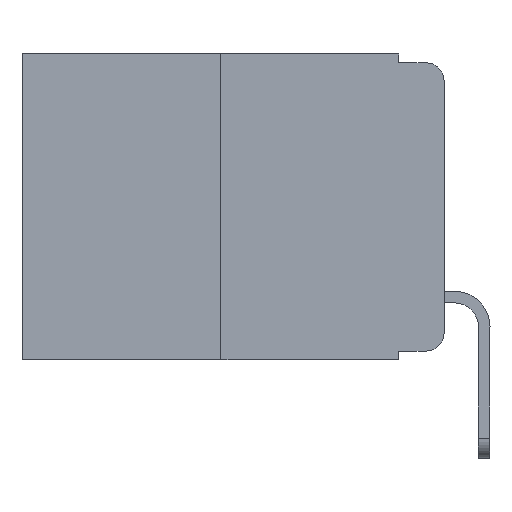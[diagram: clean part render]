
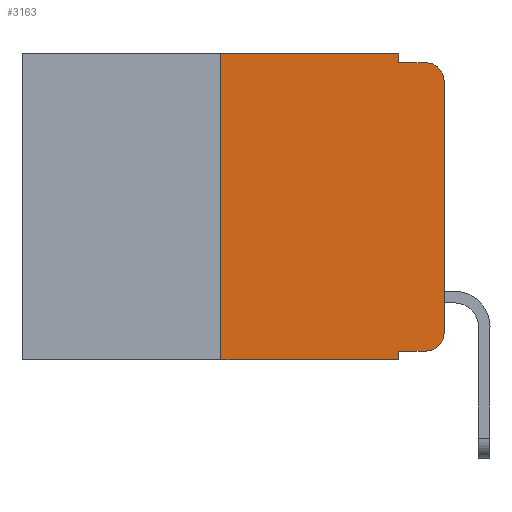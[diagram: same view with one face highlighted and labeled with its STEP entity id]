
A CAD part, left-side view. The second image highlights one B-rep face of the part: STEP entity #3163.
In plain terms, the highlighted planar face has unit normal (-1, 0, 0).
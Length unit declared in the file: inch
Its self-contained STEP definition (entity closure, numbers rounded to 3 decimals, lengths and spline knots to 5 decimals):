
#18 = DIRECTION ( 'NONE',  ( 0., 0., -1. ) ) ;
#445 = ORIENTED_EDGE ( 'NONE', *, *, #828, .F. ) ;
#467 = VERTEX_POINT ( 'NONE', #10976 ) ;
#617 = VERTEX_POINT ( 'NONE', #10006 ) ;
#828 = EDGE_CURVE ( 'NONE', #467, #3621, #6359, .T. ) ;
#1123 = EDGE_LOOP ( 'NONE', ( #1739, #3092, #2296, #1510, #1259, #13174, #13289, #445, #13529, #4531 ) ) ;
#1136 = VECTOR ( 'NONE', #7764, 39.37008 ) ;
#1208 = AXIS2_PLACEMENT_3D ( 'NONE', #9365, #3027, #10290 ) ;
#1259 = ORIENTED_EDGE ( 'NONE', *, *, #12937, .F. ) ;
#1381 = CARTESIAN_POINT ( 'NONE',  ( 0., 0.473, 0. ) ) ;
#1388 = FACE_OUTER_BOUND ( 'NONE', #1123, .T. ) ;
#1510 = ORIENTED_EDGE ( 'NONE', *, *, #7789, .F. ) ;
#1739 = ORIENTED_EDGE ( 'NONE', *, *, #2849, .T. ) ;
#1791 = LINE ( 'NONE', #5107, #4790 ) ;
#1983 = CARTESIAN_POINT ( 'NONE',  ( 0., 0.051, -0.01 ) ) ;
#2018 = EDGE_CURVE ( 'NONE', #2186, #3915, #1791, .T. ) ;
#2102 = EDGE_CURVE ( 'NONE', #617, #3561, #3253, .T. ) ;
#2186 = VERTEX_POINT ( 'NONE', #1983 ) ;
#2194 = DIRECTION ( 'NONE',  ( 0., 0., -1. ) ) ;
#2214 = DIRECTION ( 'NONE',  ( 0., -1., 0. ) ) ;
#2296 = ORIENTED_EDGE ( 'NONE', *, *, #2018, .F. ) ;
#2552 = DIRECTION ( 'NONE',  ( 0., 0., 1. ) ) ;
#2657 = EDGE_CURVE ( 'NONE', #6269, #3915, #12574, .T. ) ;
#2675 = DIRECTION ( 'NONE',  ( -1., 0., 0. ) ) ;
#2754 = EDGE_CURVE ( 'NONE', #10431, #3621, #8405, .T. ) ;
#2846 = LINE ( 'NONE', #9067, #4955 ) ;
#2849 = EDGE_CURVE ( 'NONE', #3561, #6269, #11659, .T. ) ;
#3027 = DIRECTION ( 'NONE',  ( -1., 0., 0. ) ) ;
#3092 = ORIENTED_EDGE ( 'NONE', *, *, #2657, .T. ) ;
#3163 = ADVANCED_FACE ( 'NONE', ( #1388 ), #7793, .F. ) ;
#3253 = CIRCLE ( 'NONE', #1208, 0.02 ) ;
#3314 = VECTOR ( 'NONE', #18, 39.37008 ) ;
#3561 = VERTEX_POINT ( 'NONE', #8453 ) ;
#3621 = VERTEX_POINT ( 'NONE', #13196 ) ;
#3915 = VERTEX_POINT ( 'NONE', #6934 ) ;
#4531 = ORIENTED_EDGE ( 'NONE', *, *, #2102, .T. ) ;
#4617 = LINE ( 'NONE', #11159, #9338 ) ;
#4790 = VECTOR ( 'NONE', #5153, 39.37008 ) ;
#4955 = VECTOR ( 'NONE', #6074, 39.37008 ) ;
#5042 = VERTEX_POINT ( 'NONE', #9473 ) ;
#5055 = CARTESIAN_POINT ( 'NONE',  ( 0., 0.25, 0. ) ) ;
#5107 = CARTESIAN_POINT ( 'NONE',  ( 0., 0.051, -0.01 ) ) ;
#5153 = DIRECTION ( 'NONE',  ( 0., -1., 0. ) ) ;
#5787 = CARTESIAN_POINT ( 'NONE',  ( 0., 0.473, 0. ) ) ;
#5897 = VERTEX_POINT ( 'NONE', #5055 ) ;
#6074 = DIRECTION ( 'NONE',  ( 0., -1., 0. ) ) ;
#6269 = VERTEX_POINT ( 'NONE', #8100 ) ;
#6359 = LINE ( 'NONE', #9684, #3314 ) ;
#6652 = VECTOR ( 'NONE', #2552, 39.37008 ) ;
#6779 = CARTESIAN_POINT ( 'NONE',  ( 0., 0.25, 0. ) ) ;
#6934 = CARTESIAN_POINT ( 'NONE',  ( 0., 0.02, -0.01 ) ) ;
#7169 = VECTOR ( 'NONE', #10117, 39.37008 ) ;
#7398 = DIRECTION ( 'NONE',  ( 0., 0., -1. ) ) ;
#7672 = LINE ( 'NONE', #6779, #1136 ) ;
#7764 = DIRECTION ( 'NONE',  ( 0., 0., 1. ) ) ;
#7789 = EDGE_CURVE ( 'NONE', #5042, #2186, #4617, .T. ) ;
#7793 = PLANE ( 'NONE',  #12513 ) ;
#7810 = CARTESIAN_POINT ( 'NONE',  ( 0., 0.473, -0.343 ) ) ;
#8100 = CARTESIAN_POINT ( 'NONE',  ( 0., 0., -0.03 ) ) ;
#8108 = VECTOR ( 'NONE', #2214, 39.37008 ) ;
#8405 = LINE ( 'NONE', #7810, #8108 ) ;
#8453 = CARTESIAN_POINT ( 'NONE',  ( 0., 0., -0.313 ) ) ;
#8757 = DIRECTION ( 'NONE',  ( 1., 0., 0. ) ) ;
#9067 = CARTESIAN_POINT ( 'NONE',  ( 0., 0.051, -0.333 ) ) ;
#9094 = CARTESIAN_POINT ( 'NONE',  ( 0., 0.02, -0.03 ) ) ;
#9244 = EDGE_CURVE ( 'NONE', #10431, #5897, #7672, .T. ) ;
#9338 = VECTOR ( 'NONE', #7398, 39.37008 ) ;
#9365 = CARTESIAN_POINT ( 'NONE',  ( 0., 0.02, -0.313 ) ) ;
#9473 = CARTESIAN_POINT ( 'NONE',  ( 0., 0.051, 0. ) ) ;
#9684 = CARTESIAN_POINT ( 'NONE',  ( 0., 0.051, 0. ) ) ;
#9976 = CARTESIAN_POINT ( 'NONE',  ( 0., 0., 0. ) ) ;
#10006 = CARTESIAN_POINT ( 'NONE',  ( 0., 0.02, -0.333 ) ) ;
#10057 = DIRECTION ( 'NONE',  ( 0., 0., -1. ) ) ;
#10117 = DIRECTION ( 'NONE',  ( 0., -1., 0. ) ) ;
#10290 = DIRECTION ( 'NONE',  ( 0., 0., -1. ) ) ;
#10431 = VERTEX_POINT ( 'NONE', #11420 ) ;
#10860 = EDGE_CURVE ( 'NONE', #467, #617, #2846, .T. ) ;
#10976 = CARTESIAN_POINT ( 'NONE',  ( 0., 0.051, -0.333 ) ) ;
#11159 = CARTESIAN_POINT ( 'NONE',  ( 0., 0.051, 0. ) ) ;
#11420 = CARTESIAN_POINT ( 'NONE',  ( 0., 0.25, -0.343 ) ) ;
#11659 = LINE ( 'NONE', #9976, #6652 ) ;
#12356 = AXIS2_PLACEMENT_3D ( 'NONE', #9094, #2675, #10057 ) ;
#12513 = AXIS2_PLACEMENT_3D ( 'NONE', #5787, #8757, #2194 ) ;
#12574 = CIRCLE ( 'NONE', #12356, 0.02 ) ;
#12937 = EDGE_CURVE ( 'NONE', #5897, #5042, #13648, .T. ) ;
#13174 = ORIENTED_EDGE ( 'NONE', *, *, #9244, .F. ) ;
#13196 = CARTESIAN_POINT ( 'NONE',  ( 0., 0.051, -0.343 ) ) ;
#13289 = ORIENTED_EDGE ( 'NONE', *, *, #2754, .T. ) ;
#13529 = ORIENTED_EDGE ( 'NONE', *, *, #10860, .T. ) ;
#13648 = LINE ( 'NONE', #1381, #7169 ) ;
